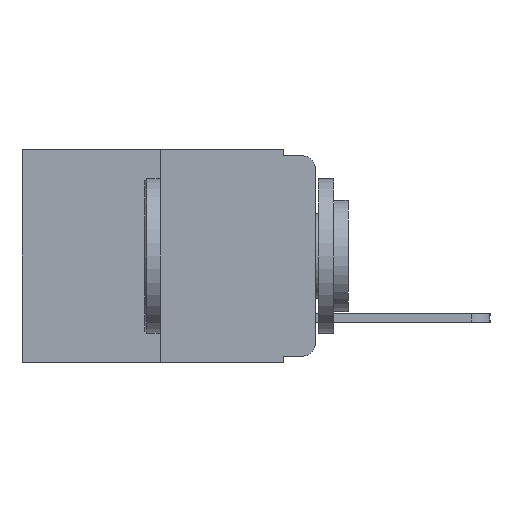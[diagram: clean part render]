
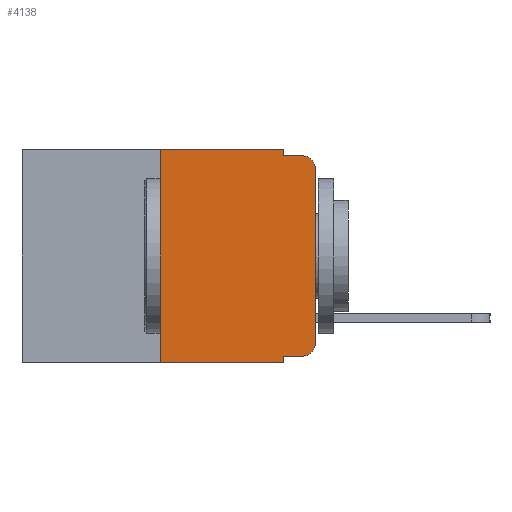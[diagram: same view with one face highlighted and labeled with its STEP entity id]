
A CAD part, left-side view. The second image highlights one B-rep face of the part: STEP entity #4138.
In plain terms, the highlighted planar face has unit normal (-1, 0, 0).
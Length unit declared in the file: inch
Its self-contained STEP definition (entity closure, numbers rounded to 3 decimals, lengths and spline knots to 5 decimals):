
#83 = CARTESIAN_POINT ( 'NONE',  ( 0., 0.051, -0.343 ) ) ;
#200 = VERTEX_POINT ( 'NONE', #1727 ) ;
#272 = CARTESIAN_POINT ( 'NONE',  ( 0., 0., -0.313 ) ) ;
#821 = VERTEX_POINT ( 'NONE', #3080 ) ;
#1076 = CIRCLE ( 'NONE', #11926, 0.02 ) ;
#1232 = CARTESIAN_POINT ( 'NONE',  ( 0., 0.051, 0. ) ) ;
#1315 = CARTESIAN_POINT ( 'NONE',  ( 0., 0.051, -0.01 ) ) ;
#1317 = VECTOR ( 'NONE', #7077, 39.37008 ) ;
#1545 = ORIENTED_EDGE ( 'NONE', *, *, #2847, .T. ) ;
#1727 = CARTESIAN_POINT ( 'NONE',  ( 0., 0.051, 0. ) ) ;
#1759 = FACE_OUTER_BOUND ( 'NONE', #8725, .T. ) ;
#1841 = ORIENTED_EDGE ( 'NONE', *, *, #3837, .T. ) ;
#2102 = AXIS2_PLACEMENT_3D ( 'NONE', #11260, #12491, #2717 ) ;
#2495 = CARTESIAN_POINT ( 'NONE',  ( 0., 0.02, -0.313 ) ) ;
#2573 = ORIENTED_EDGE ( 'NONE', *, *, #5732, .F. ) ;
#2589 = DIRECTION ( 'NONE',  ( -1., 0., 0. ) ) ;
#2717 = DIRECTION ( 'NONE',  ( 0., 0., -1. ) ) ;
#2847 = EDGE_CURVE ( 'NONE', #11474, #11089, #5733, .T. ) ;
#2985 = VECTOR ( 'NONE', #10564, 39.37008 ) ;
#3080 = CARTESIAN_POINT ( 'NONE',  ( 0., 0.25, -0.343 ) ) ;
#3117 = ORIENTED_EDGE ( 'NONE', *, *, #6175, .F. ) ;
#3322 = VECTOR ( 'NONE', #9177, 39.37008 ) ;
#3498 = ORIENTED_EDGE ( 'NONE', *, *, #11406, .F. ) ;
#3837 = EDGE_CURVE ( 'NONE', #11089, #3994, #10460, .T. ) ;
#3913 = EDGE_CURVE ( 'NONE', #821, #5415, #9086, .T. ) ;
#3958 = VERTEX_POINT ( 'NONE', #6712 ) ;
#3994 = VERTEX_POINT ( 'NONE', #5115 ) ;
#4006 = VERTEX_POINT ( 'NONE', #7396 ) ;
#4053 = ORIENTED_EDGE ( 'NONE', *, *, #3913, .F. ) ;
#4138 = ADVANCED_FACE ( 'NONE', ( #1759 ), #11022, .F. ) ;
#4265 = VERTEX_POINT ( 'NONE', #83 ) ;
#4343 = ORIENTED_EDGE ( 'NONE', *, *, #6389, .T. ) ;
#4401 = VECTOR ( 'NONE', #5794, 39.37008 ) ;
#4416 = VECTOR ( 'NONE', #6875, 39.37008 ) ;
#4600 = VERTEX_POINT ( 'NONE', #1315 ) ;
#4671 = ORIENTED_EDGE ( 'NONE', *, *, #8900, .F. ) ;
#5115 = CARTESIAN_POINT ( 'NONE',  ( 0., 0.02, -0.01 ) ) ;
#5415 = VERTEX_POINT ( 'NONE', #7441 ) ;
#5626 = ORIENTED_EDGE ( 'NONE', *, *, #7228, .T. ) ;
#5732 = EDGE_CURVE ( 'NONE', #4600, #3994, #7113, .T. ) ;
#5733 = LINE ( 'NONE', #12947, #3322 ) ;
#5794 = DIRECTION ( 'NONE',  ( 0., 0., -1. ) ) ;
#5900 = CARTESIAN_POINT ( 'NONE',  ( 0., 0.051, 0. ) ) ;
#6049 = ORIENTED_EDGE ( 'NONE', *, *, #7935, .T. ) ;
#6068 = CARTESIAN_POINT ( 'NONE',  ( 0., 0.02, -0.03 ) ) ;
#6175 = EDGE_CURVE ( 'NONE', #200, #4600, #7095, .T. ) ;
#6335 = VECTOR ( 'NONE', #7904, 39.37008 ) ;
#6389 = EDGE_CURVE ( 'NONE', #821, #4265, #6918, .T. ) ;
#6712 = CARTESIAN_POINT ( 'NONE',  ( 0., 0.02, -0.333 ) ) ;
#6875 = DIRECTION ( 'NONE',  ( 0., -1., 0. ) ) ;
#6918 = LINE ( 'NONE', #8477, #1317 ) ;
#7077 = DIRECTION ( 'NONE',  ( 0., -1., 0. ) ) ;
#7095 = LINE ( 'NONE', #5900, #4401 ) ;
#7113 = LINE ( 'NONE', #12155, #4416 ) ;
#7228 = EDGE_CURVE ( 'NONE', #4006, #3958, #12428, .T. ) ;
#7231 = VECTOR ( 'NONE', #12185, 39.37008 ) ;
#7396 = CARTESIAN_POINT ( 'NONE',  ( 0., 0.051, -0.333 ) ) ;
#7441 = CARTESIAN_POINT ( 'NONE',  ( 0., 0.25, 0. ) ) ;
#7494 = AXIS2_PLACEMENT_3D ( 'NONE', #6068, #10979, #10963 ) ;
#7687 = DIRECTION ( 'NONE',  ( 0., -1., 0. ) ) ;
#7904 = DIRECTION ( 'NONE',  ( 0., 0., 1. ) ) ;
#7935 = EDGE_CURVE ( 'NONE', #3958, #11474, #1076, .T. ) ;
#8277 = CARTESIAN_POINT ( 'NONE',  ( 0., 0., -0.03 ) ) ;
#8477 = CARTESIAN_POINT ( 'NONE',  ( 0., 0.473, -0.343 ) ) ;
#8725 = EDGE_LOOP ( 'NONE', ( #1545, #1841, #2573, #3117, #3498, #4053, #4343, #4671, #5626, #6049 ) ) ;
#8900 = EDGE_CURVE ( 'NONE', #4006, #4265, #11067, .T. ) ;
#9086 = LINE ( 'NONE', #9506, #6335 ) ;
#9177 = DIRECTION ( 'NONE',  ( 0., 0., 1. ) ) ;
#9506 = CARTESIAN_POINT ( 'NONE',  ( 0., 0.25, 0. ) ) ;
#9752 = LINE ( 'NONE', #10672, #11967 ) ;
#10460 = CIRCLE ( 'NONE', #7494, 0.02 ) ;
#10564 = DIRECTION ( 'NONE',  ( 0., 0., -1. ) ) ;
#10672 = CARTESIAN_POINT ( 'NONE',  ( 0., 0.473, 0. ) ) ;
#10963 = DIRECTION ( 'NONE',  ( 0., 0., -1. ) ) ;
#10979 = DIRECTION ( 'NONE',  ( -1., 0., 0. ) ) ;
#11022 = PLANE ( 'NONE',  #2102 ) ;
#11067 = LINE ( 'NONE', #1232, #2985 ) ;
#11089 = VERTEX_POINT ( 'NONE', #8277 ) ;
#11260 = CARTESIAN_POINT ( 'NONE',  ( 0., 0.473, 0. ) ) ;
#11406 = EDGE_CURVE ( 'NONE', #5415, #200, #9752, .T. ) ;
#11417 = DIRECTION ( 'NONE',  ( 0., 0., -1. ) ) ;
#11474 = VERTEX_POINT ( 'NONE', #272 ) ;
#11926 = AXIS2_PLACEMENT_3D ( 'NONE', #2495, #2589, #11417 ) ;
#11967 = VECTOR ( 'NONE', #7687, 39.37008 ) ;
#12155 = CARTESIAN_POINT ( 'NONE',  ( 0., 0.051, -0.01 ) ) ;
#12185 = DIRECTION ( 'NONE',  ( 0., -1., 0. ) ) ;
#12428 = LINE ( 'NONE', #13058, #7231 ) ;
#12491 = DIRECTION ( 'NONE',  ( 1., 0., 0. ) ) ;
#12947 = CARTESIAN_POINT ( 'NONE',  ( 0., 0., 0. ) ) ;
#13058 = CARTESIAN_POINT ( 'NONE',  ( 0., 0.051, -0.333 ) ) ;
